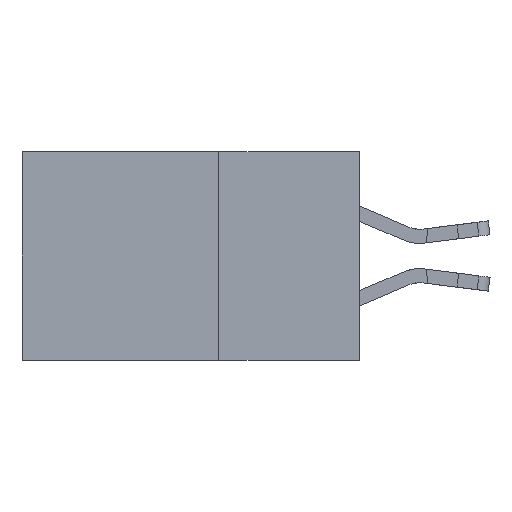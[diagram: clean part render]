
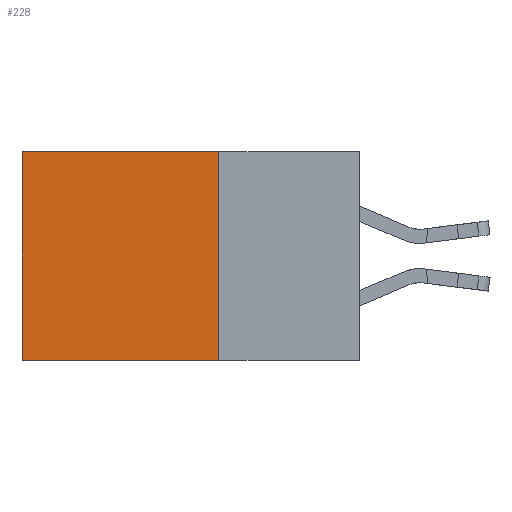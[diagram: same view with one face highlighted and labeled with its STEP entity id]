
A CAD part, left-side view. The second image highlights one B-rep face of the part: STEP entity #228.
In plain terms, the highlighted planar face has unit normal (-1, 0, 0).
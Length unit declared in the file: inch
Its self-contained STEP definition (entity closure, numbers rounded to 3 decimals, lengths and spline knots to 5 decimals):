
#228 = ADVANCED_FACE ( 'NONE', ( #6534 ), #10954, .F. ) ;
#1912 = CARTESIAN_POINT ( 'NONE',  ( 0.2875, 0.6, 0. ) ) ;
#2005 = CARTESIAN_POINT ( 'NONE',  ( 0.2875, 0.25, 0. ) ) ;
#2094 = DIRECTION ( 'NONE',  ( 0., 1., 0. ) ) ;
#2787 = CARTESIAN_POINT ( 'NONE',  ( 0.2875, 0.25, 0. ) ) ;
#2845 = ORIENTED_EDGE ( 'NONE', *, *, #10470, .T. ) ;
#3267 = DIRECTION ( 'NONE',  ( 0., 0., -1. ) ) ;
#3278 = DIRECTION ( 'NONE',  ( 0., 0., -1. ) ) ;
#3900 = VERTEX_POINT ( 'NONE', #9191 ) ;
#4033 = AXIS2_PLACEMENT_3D ( 'NONE', #2005, #14450, #3267 ) ;
#4181 = DIRECTION ( 'NONE',  ( 0., 1., 0. ) ) ;
#4277 = DIRECTION ( 'NONE',  ( 0., 0., -1. ) ) ;
#4303 = VECTOR ( 'NONE', #4181, 39.37008 ) ;
#5205 = LINE ( 'NONE', #2787, #4303 ) ;
#5560 = VERTEX_POINT ( 'NONE', #11187 ) ;
#5766 = VECTOR ( 'NONE', #4277, 39.37008 ) ;
#6534 = FACE_OUTER_BOUND ( 'NONE', #10391, .T. ) ;
#7069 = VECTOR ( 'NONE', #3278, 39.37008 ) ;
#7580 = EDGE_CURVE ( 'NONE', #17360, #3900, #16178, .T. ) ;
#7692 = LINE ( 'NONE', #8993, #14478 ) ;
#8451 = CARTESIAN_POINT ( 'NONE',  ( 0.2875, 0.25, 0. ) ) ;
#8993 = CARTESIAN_POINT ( 'NONE',  ( 0.2875, 0.25, -0.37 ) ) ;
#9191 = CARTESIAN_POINT ( 'NONE',  ( 0.2875, 0.25, -0.37 ) ) ;
#9422 = ORIENTED_EDGE ( 'NONE', *, *, #7580, .F. ) ;
#10289 = LINE ( 'NONE', #1912, #7069 ) ;
#10391 = EDGE_LOOP ( 'NONE', ( #16635, #13969, #9422, #2845 ) ) ;
#10470 = EDGE_CURVE ( 'NONE', #17360, #11497, #5205, .T. ) ;
#10954 = PLANE ( 'NONE',  #4033 ) ;
#11187 = CARTESIAN_POINT ( 'NONE',  ( 0.2875, 0.6, -0.37 ) ) ;
#11497 = VERTEX_POINT ( 'NONE', #12071 ) ;
#12071 = CARTESIAN_POINT ( 'NONE',  ( 0.2875, 0.6, 0. ) ) ;
#12519 = EDGE_CURVE ( 'NONE', #11497, #5560, #10289, .T. ) ;
#13149 = EDGE_CURVE ( 'NONE', #3900, #5560, #7692, .T. ) ;
#13969 = ORIENTED_EDGE ( 'NONE', *, *, #13149, .F. ) ;
#14450 = DIRECTION ( 'NONE',  ( 1., 0., 0. ) ) ;
#14478 = VECTOR ( 'NONE', #2094, 39.37008 ) ;
#14531 = CARTESIAN_POINT ( 'NONE',  ( 0.2875, 0.25, 0. ) ) ;
#16178 = LINE ( 'NONE', #8451, #5766 ) ;
#16635 = ORIENTED_EDGE ( 'NONE', *, *, #12519, .T. ) ;
#17360 = VERTEX_POINT ( 'NONE', #14531 ) ;
